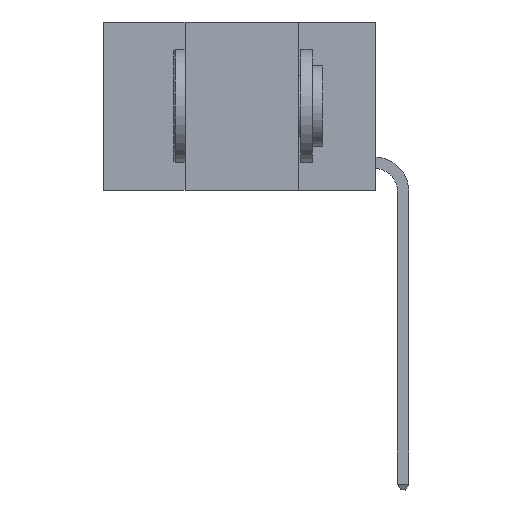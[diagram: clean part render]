
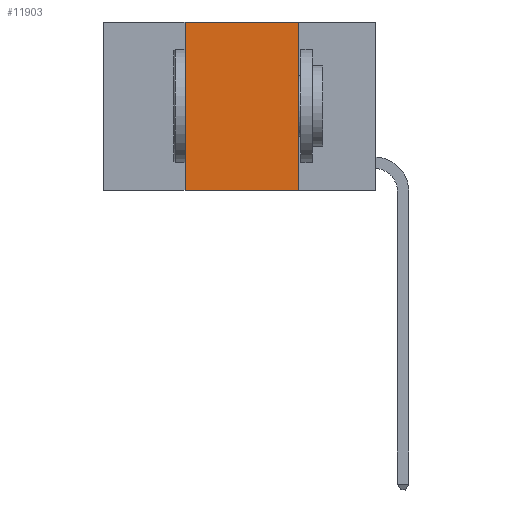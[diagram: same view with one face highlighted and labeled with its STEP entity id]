
A CAD part, left-side view. The second image highlights one B-rep face of the part: STEP entity #11903.
In plain terms, the highlighted planar face has unit normal (-1, 0, 0).
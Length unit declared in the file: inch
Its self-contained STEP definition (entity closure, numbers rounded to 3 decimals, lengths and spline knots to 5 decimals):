
#1191 = ORIENTED_EDGE ( 'NONE', *, *, #19865, .F. ) ;
#1353 = VERTEX_POINT ( 'NONE', #2696 ) ;
#1490 = LINE ( 'NONE', #23938, #6343 ) ;
#2074 = VECTOR ( 'NONE', #24184, 39.37008 ) ;
#2280 = DIRECTION ( 'NONE',  ( 0., -1., 0. ) ) ;
#2696 = CARTESIAN_POINT ( 'NONE',  ( 0., 0.17, -0.37 ) ) ;
#3219 = VERTEX_POINT ( 'NONE', #3775 ) ;
#3687 = EDGE_LOOP ( 'NONE', ( #26954, #18682, #1191, #17994 ) ) ;
#3775 = CARTESIAN_POINT ( 'NONE',  ( 0., 0.42, -0.37 ) ) ;
#5042 = DIRECTION ( 'NONE',  ( 0., 0., -1. ) ) ;
#5346 = LINE ( 'NONE', #25517, #29439 ) ;
#6343 = VECTOR ( 'NONE', #26238, 39.37008 ) ;
#7158 = VECTOR ( 'NONE', #2280, 39.37008 ) ;
#8575 = AXIS2_PLACEMENT_3D ( 'NONE', #23785, #19184, #5042 ) ;
#9085 = CARTESIAN_POINT ( 'NONE',  ( 0., 0.17, 0. ) ) ;
#10113 = CARTESIAN_POINT ( 'NONE',  ( 0., 0.6, -0.37 ) ) ;
#11679 = VERTEX_POINT ( 'NONE', #9085 ) ;
#11903 = ADVANCED_FACE ( 'NONE', ( #29877 ), #14448, .F. ) ;
#11998 = EDGE_CURVE ( 'NONE', #3219, #1353, #20897, .T. ) ;
#12980 = EDGE_CURVE ( 'NONE', #11679, #1353, #5346, .T. ) ;
#14448 = PLANE ( 'NONE',  #8575 ) ;
#15710 = VERTEX_POINT ( 'NONE', #29974 ) ;
#17994 = ORIENTED_EDGE ( 'NONE', *, *, #11998, .T. ) ;
#18682 = ORIENTED_EDGE ( 'NONE', *, *, #24087, .F. ) ;
#19184 = DIRECTION ( 'NONE',  ( 1., 0., 0. ) ) ;
#19865 = EDGE_CURVE ( 'NONE', #3219, #15710, #1490, .T. ) ;
#20897 = LINE ( 'NONE', #10113, #2074 ) ;
#23222 = DIRECTION ( 'NONE',  ( 0., 0., -1. ) ) ;
#23785 = CARTESIAN_POINT ( 'NONE',  ( 0., 0.6, 0. ) ) ;
#23938 = CARTESIAN_POINT ( 'NONE',  ( 0., 0.42, 0. ) ) ;
#24087 = EDGE_CURVE ( 'NONE', #15710, #11679, #25846, .T. ) ;
#24184 = DIRECTION ( 'NONE',  ( 0., -1., 0. ) ) ;
#25517 = CARTESIAN_POINT ( 'NONE',  ( 0., 0.17, 0. ) ) ;
#25846 = LINE ( 'NONE', #30264, #7158 ) ;
#26238 = DIRECTION ( 'NONE',  ( 0., 0., 1. ) ) ;
#26954 = ORIENTED_EDGE ( 'NONE', *, *, #12980, .F. ) ;
#29439 = VECTOR ( 'NONE', #23222, 39.37008 ) ;
#29877 = FACE_OUTER_BOUND ( 'NONE', #3687, .T. ) ;
#29974 = CARTESIAN_POINT ( 'NONE',  ( 0., 0.42, 0. ) ) ;
#30264 = CARTESIAN_POINT ( 'NONE',  ( 0., 0.6, 0. ) ) ;
